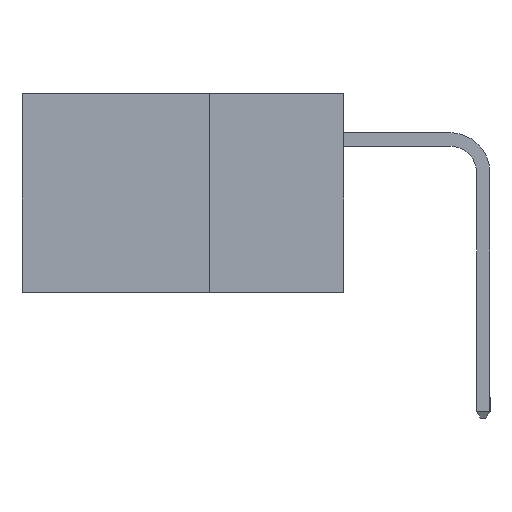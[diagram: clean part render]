
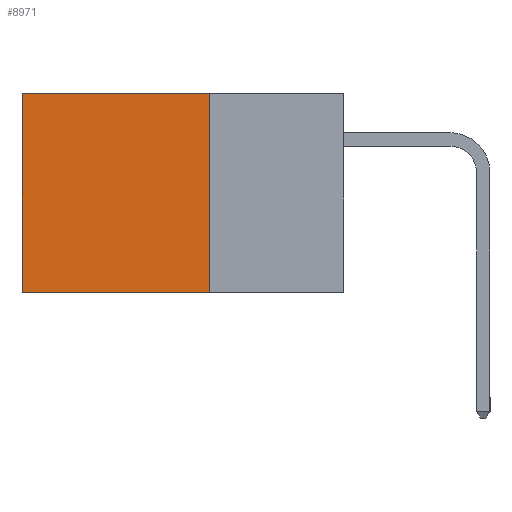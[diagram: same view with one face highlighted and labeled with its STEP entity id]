
A CAD part, left-side view. The second image highlights one B-rep face of the part: STEP entity #8971.
In plain terms, the highlighted planar face has unit normal (-1, 0, 0).
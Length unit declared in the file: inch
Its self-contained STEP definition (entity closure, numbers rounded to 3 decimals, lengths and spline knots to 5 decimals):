
#1141 = DIRECTION ( 'NONE',  ( 1., 0., 0. ) ) ;
#3089 = DIRECTION ( 'NONE',  ( 0., 0., -1. ) ) ;
#3631 = VECTOR ( 'NONE', #7683, 39.37008 ) ;
#4287 = CARTESIAN_POINT ( 'NONE',  ( 0.2615, 0.25, 0. ) ) ;
#4583 = CARTESIAN_POINT ( 'NONE',  ( 0.2615, 0.25, -0.37 ) ) ;
#5260 = EDGE_CURVE ( 'NONE', #16234, #6504, #16482, .T. ) ;
#5870 = DIRECTION ( 'NONE',  ( 0., 1., 0. ) ) ;
#6504 = VERTEX_POINT ( 'NONE', #7504 ) ;
#7495 = VECTOR ( 'NONE', #3089, 39.37008 ) ;
#7504 = CARTESIAN_POINT ( 'NONE',  ( 0.2615, 0.6, -0.37 ) ) ;
#7683 = DIRECTION ( 'NONE',  ( 0., 1., 0. ) ) ;
#7738 = CARTESIAN_POINT ( 'NONE',  ( 0.2615, 0.6, -0.37 ) ) ;
#7922 = EDGE_LOOP ( 'NONE', ( #16025, #14399, #10430, #18040 ) ) ;
#8106 = EDGE_CURVE ( 'NONE', #10146, #16234, #16091, .T. ) ;
#8208 = AXIS2_PLACEMENT_3D ( 'NONE', #10474, #1141, #12032 ) ;
#8264 = CARTESIAN_POINT ( 'NONE',  ( 0.2615, 0.25, -0.37 ) ) ;
#8971 = ADVANCED_FACE ( 'NONE', ( #16540 ), #19632, .F. ) ;
#9652 = EDGE_CURVE ( 'NONE', #10146, #10958, #19368, .T. ) ;
#10146 = VERTEX_POINT ( 'NONE', #19394 ) ;
#10430 = ORIENTED_EDGE ( 'NONE', *, *, #8106, .F. ) ;
#10474 = CARTESIAN_POINT ( 'NONE',  ( 0.2615, 0.25, -0.37 ) ) ;
#10958 = VERTEX_POINT ( 'NONE', #14658 ) ;
#11630 = LINE ( 'NONE', #7738, #7495 ) ;
#12032 = DIRECTION ( 'NONE',  ( 0., 0., -1. ) ) ;
#12035 = VECTOR ( 'NONE', #14731, 39.37008 ) ;
#14399 = ORIENTED_EDGE ( 'NONE', *, *, #5260, .F. ) ;
#14438 = EDGE_CURVE ( 'NONE', #10958, #6504, #11630, .T. ) ;
#14658 = CARTESIAN_POINT ( 'NONE',  ( 0.2615, 0.6, 0. ) ) ;
#14731 = DIRECTION ( 'NONE',  ( 0., 0., -1. ) ) ;
#15387 = CARTESIAN_POINT ( 'NONE',  ( 0.2615, 0.25, -0.37 ) ) ;
#15786 = VECTOR ( 'NONE', #5870, 39.37008 ) ;
#16025 = ORIENTED_EDGE ( 'NONE', *, *, #14438, .T. ) ;
#16091 = LINE ( 'NONE', #8264, #12035 ) ;
#16234 = VERTEX_POINT ( 'NONE', #4583 ) ;
#16482 = LINE ( 'NONE', #15387, #3631 ) ;
#16540 = FACE_OUTER_BOUND ( 'NONE', #7922, .T. ) ;
#18040 = ORIENTED_EDGE ( 'NONE', *, *, #9652, .T. ) ;
#19368 = LINE ( 'NONE', #4287, #15786 ) ;
#19394 = CARTESIAN_POINT ( 'NONE',  ( 0.2615, 0.25, 0. ) ) ;
#19632 = PLANE ( 'NONE',  #8208 ) ;
